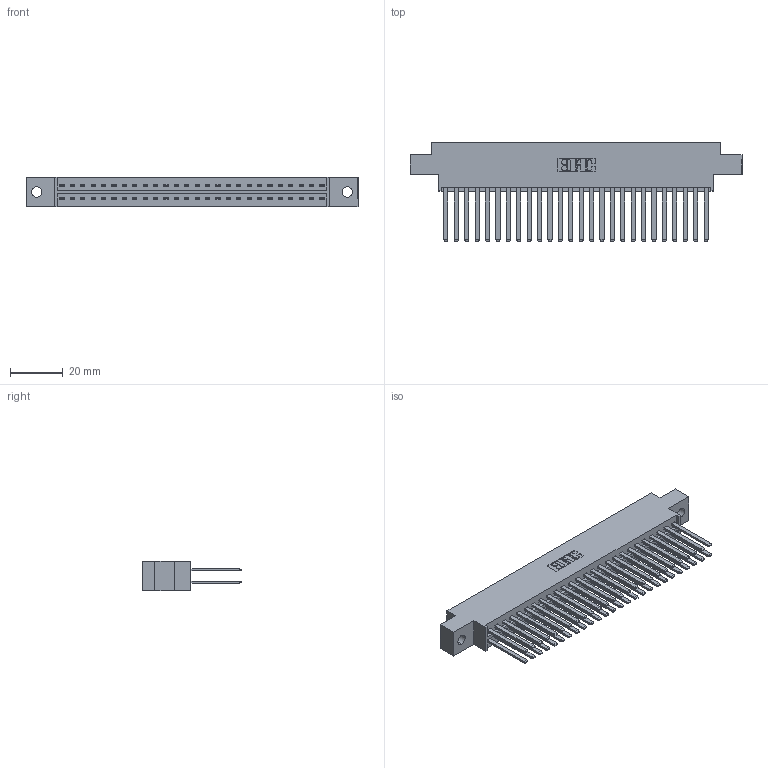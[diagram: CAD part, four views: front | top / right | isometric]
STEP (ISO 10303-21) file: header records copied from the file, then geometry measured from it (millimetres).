
FILE_DESCRIPTION (( 'STEP AP203' ), '1' );
FILE_NAME ('336-052-541-804.STEP', '2020-08-08T00:15:21', ( '' ), ( '' ), 'SwSTEP 2.0', 'SolidWorks 2020', '' );
FILE_SCHEMA (( 'CONFIG_CONTROL_DESIGN' ));
Length unit declared in the file: inch
Products named in the file (3): 336 Part_Offset - .156 Dia - TH; 336-052-541-804; 336-290-001_336-290-541
Assembly tree (53 placements, depth 2):
  336-052-541-804
    336 Part_Offset - .156 Dia - TH
    336-290-001_336-290-541  x52
Bounding box: 126.42 x 37.34 x 11.1 mm (x, y, z)
Volume: 18922.4 mm3; surface area: 23780.7 mm2
Topology: 53 solids, 53 shells, 2302 faces, 6927 edges, 4582 vertices
Faces by surface type: plane 1426, cylinder 876
Entity records: 22082 total; most frequent: CARTESIAN_POINT 3817, ORIENTED_EDGE 3654, DIRECTION 3179, EDGE_CURVE 1827, VECTOR 1695, LINE 1695, VERTEX_POINT 1216, AXIS2_PLACEMENT_3D 742
